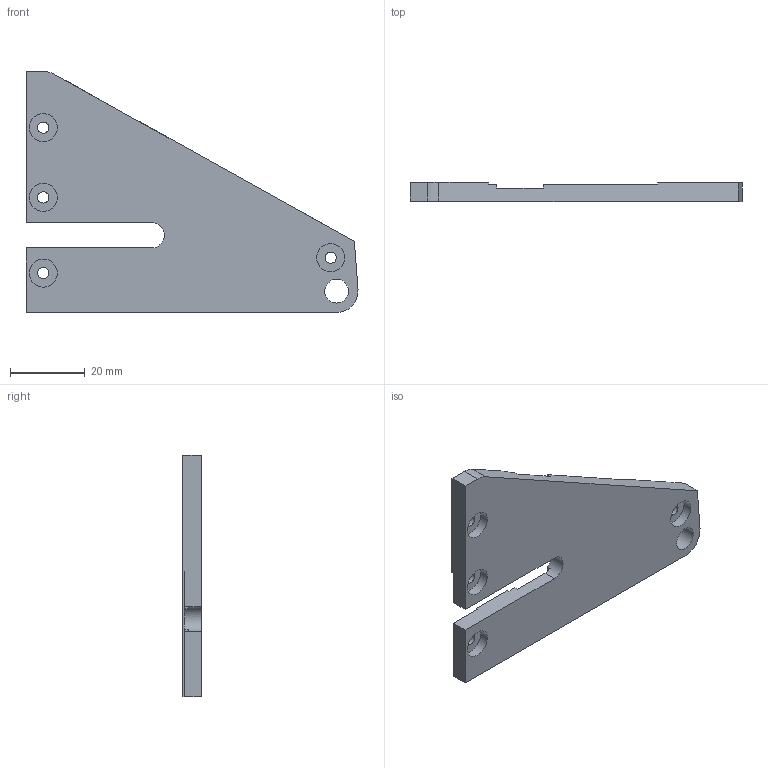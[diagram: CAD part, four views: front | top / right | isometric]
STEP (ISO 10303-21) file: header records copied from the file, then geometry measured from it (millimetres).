
FILE_DESCRIPTION (( 'STEP AP214' ), '1' );
FILE_NAME ('JT_Mag_Well_Left.step', '2016-01-30T20:06:03', ( 'WarFairy' ), ( '' ), 'SwSTEP 2.0', 'SolidWorks 2015', '' );
FILE_SCHEMA (( 'AUTOMOTIVE_DESIGN' ));
Length unit declared in the file: millimetre
Products named in the file (1): JT_Mag_Well_Left
Bounding box: 88.63 x 5 x 64.36 mm (x, y, z)
Volume: 15541.7 mm3; surface area: 9118.6 mm2
Topology: 1 solids, 1 shells, 45 faces, 123 edges, 84 vertices
Faces by surface type: plane 33, cylinder 12
Full cylindrical faces by diameter (mm): 3 x4, 6.35 x1, 7.5 x4
Entity records: 1386 total; most frequent: CARTESIAN_POINT 232, DIRECTION 226, ORIENTED_EDGE 216, EDGE_CURVE 108, VECTOR 82, LINE 82, VERTEX_POINT 78, AXIS2_PLACEMENT_3D 72
